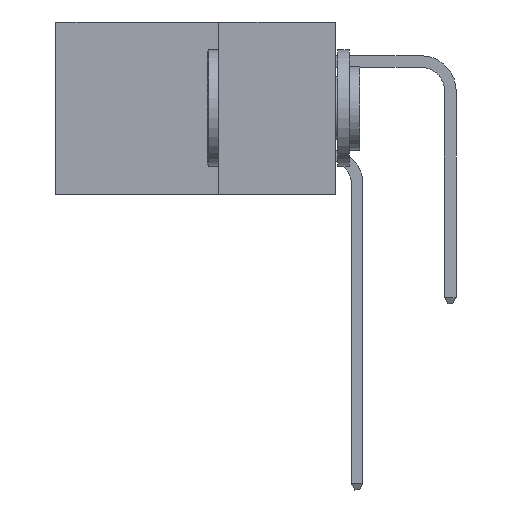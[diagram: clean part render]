
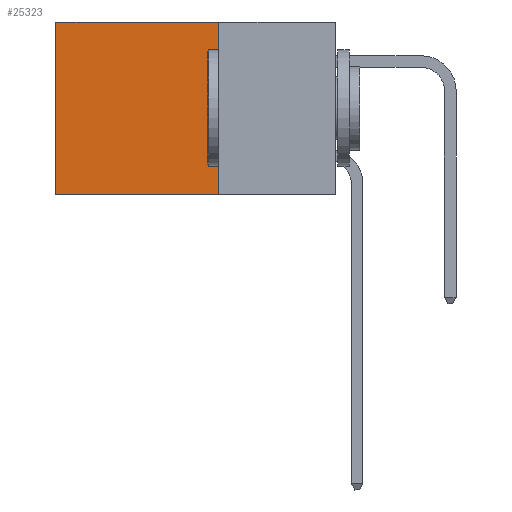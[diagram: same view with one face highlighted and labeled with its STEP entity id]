
A CAD part, left-side view. The second image highlights one B-rep face of the part: STEP entity #25323.
In plain terms, the highlighted planar face has unit normal (-1, 0, 0).
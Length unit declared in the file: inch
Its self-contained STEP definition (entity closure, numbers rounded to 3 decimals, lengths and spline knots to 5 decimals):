
#1074 = VERTEX_POINT ( 'NONE', #10262 ) ;
#1206 = LINE ( 'NONE', #23381, #22344 ) ;
#3324 = VERTEX_POINT ( 'NONE', #17740 ) ;
#3760 = VECTOR ( 'NONE', #16536, 39.37008 ) ;
#4503 = ORIENTED_EDGE ( 'NONE', *, *, #9655, .T. ) ;
#4700 = DIRECTION ( 'NONE',  ( 0., 0., -1. ) ) ;
#6144 = CARTESIAN_POINT ( 'NONE',  ( 0.2875, 0.6, 0. ) ) ;
#6774 = VERTEX_POINT ( 'NONE', #10831 ) ;
#9044 = EDGE_CURVE ( 'NONE', #9886, #6774, #20411, .T. ) ;
#9655 = EDGE_CURVE ( 'NONE', #3324, #6774, #12948, .T. ) ;
#9886 = VERTEX_POINT ( 'NONE', #15272 ) ;
#9931 = EDGE_CURVE ( 'NONE', #1074, #3324, #20361, .T. ) ;
#10262 = CARTESIAN_POINT ( 'NONE',  ( 0.2875, 0.25, 0. ) ) ;
#10831 = CARTESIAN_POINT ( 'NONE',  ( 0.2875, 0.6, -0.37 ) ) ;
#12749 = FACE_OUTER_BOUND ( 'NONE', #17866, .T. ) ;
#12948 = LINE ( 'NONE', #6144, #14589 ) ;
#14530 = CARTESIAN_POINT ( 'NONE',  ( 0.2875, 0.25, -0.37 ) ) ;
#14549 = DIRECTION ( 'NONE',  ( 0., 0., -1. ) ) ;
#14589 = VECTOR ( 'NONE', #4700, 39.37008 ) ;
#15176 = DIRECTION ( 'NONE',  ( 0., 0., -1. ) ) ;
#15272 = CARTESIAN_POINT ( 'NONE',  ( 0.2875, 0.25, -0.37 ) ) ;
#16536 = DIRECTION ( 'NONE',  ( 0., 1., 0. ) ) ;
#16642 = VECTOR ( 'NONE', #18628, 39.37008 ) ;
#17169 = CARTESIAN_POINT ( 'NONE',  ( 0.2875, 0.25, 0. ) ) ;
#17740 = CARTESIAN_POINT ( 'NONE',  ( 0.2875, 0.6, 0. ) ) ;
#17866 = EDGE_LOOP ( 'NONE', ( #4503, #27775, #18017, #23944 ) ) ;
#17953 = CARTESIAN_POINT ( 'NONE',  ( 0.2875, 0.25, 0. ) ) ;
#18017 = ORIENTED_EDGE ( 'NONE', *, *, #27541, .F. ) ;
#18628 = DIRECTION ( 'NONE',  ( 0., 1., 0. ) ) ;
#19880 = AXIS2_PLACEMENT_3D ( 'NONE', #17169, #27933, #15176 ) ;
#20361 = LINE ( 'NONE', #17953, #16642 ) ;
#20411 = LINE ( 'NONE', #14530, #3760 ) ;
#22344 = VECTOR ( 'NONE', #14549, 39.37008 ) ;
#23381 = CARTESIAN_POINT ( 'NONE',  ( 0.2875, 0.25, 0. ) ) ;
#23944 = ORIENTED_EDGE ( 'NONE', *, *, #9931, .T. ) ;
#25323 = ADVANCED_FACE ( 'NONE', ( #12749 ), #25885, .F. ) ;
#25885 = PLANE ( 'NONE',  #19880 ) ;
#27541 = EDGE_CURVE ( 'NONE', #1074, #9886, #1206, .T. ) ;
#27775 = ORIENTED_EDGE ( 'NONE', *, *, #9044, .F. ) ;
#27933 = DIRECTION ( 'NONE',  ( 1., 0., 0. ) ) ;
